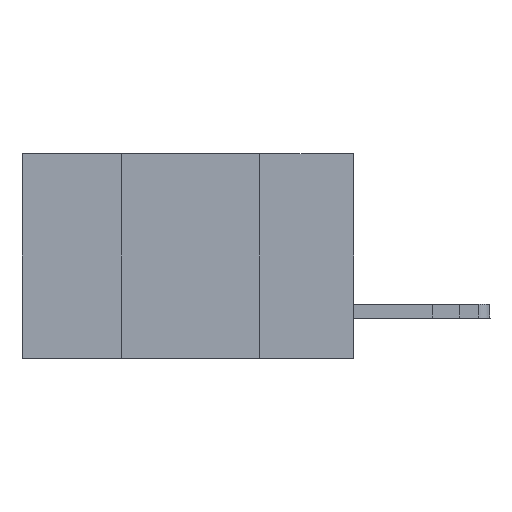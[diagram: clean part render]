
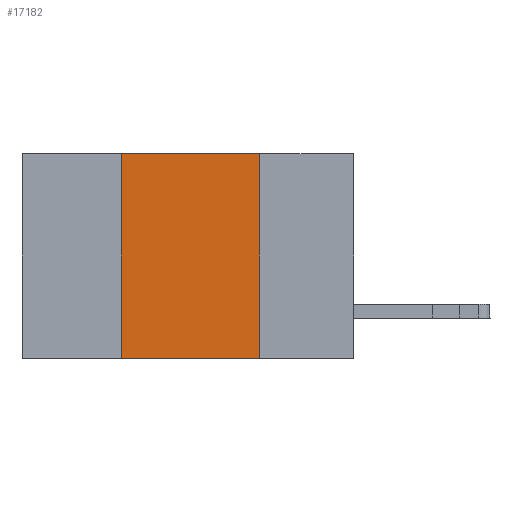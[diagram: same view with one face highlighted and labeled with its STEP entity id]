
A CAD part, left-side view. The second image highlights one B-rep face of the part: STEP entity #17182.
In plain terms, the highlighted planar face has unit normal (-1, 0, 0).
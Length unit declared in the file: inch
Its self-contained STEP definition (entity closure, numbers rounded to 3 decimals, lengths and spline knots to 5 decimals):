
#90 = CARTESIAN_POINT ( 'NONE',  ( 0., 0.42, 0. ) ) ;
#2150 = LINE ( 'NONE', #21750, #16067 ) ;
#2595 = DIRECTION ( 'NONE',  ( 0., -1., 0. ) ) ;
#3622 = ORIENTED_EDGE ( 'NONE', *, *, #23230, .F. ) ;
#3762 = AXIS2_PLACEMENT_3D ( 'NONE', #12570, #19631, #21415 ) ;
#4135 = ORIENTED_EDGE ( 'NONE', *, *, #12864, .F. ) ;
#4386 = VERTEX_POINT ( 'NONE', #21179 ) ;
#4761 = CARTESIAN_POINT ( 'NONE',  ( 0., 0.42, -0.37 ) ) ;
#5532 = DIRECTION ( 'NONE',  ( 0., 0., -1. ) ) ;
#6596 = LINE ( 'NONE', #8507, #18741 ) ;
#6712 = VERTEX_POINT ( 'NONE', #90 ) ;
#7334 = CARTESIAN_POINT ( 'NONE',  ( 0., 0.17, 0. ) ) ;
#8098 = LINE ( 'NONE', #17040, #13176 ) ;
#8507 = CARTESIAN_POINT ( 'NONE',  ( 0., 0.42, 0. ) ) ;
#8813 = VECTOR ( 'NONE', #5532, 39.37008 ) ;
#10406 = ORIENTED_EDGE ( 'NONE', *, *, #21756, .T. ) ;
#10437 = PLANE ( 'NONE',  #3762 ) ;
#11004 = ORIENTED_EDGE ( 'NONE', *, *, #22973, .F. ) ;
#11367 = EDGE_LOOP ( 'NONE', ( #11004, #4135, #3622, #10406 ) ) ;
#12065 = VERTEX_POINT ( 'NONE', #20813 ) ;
#12570 = CARTESIAN_POINT ( 'NONE',  ( 0., 0.6, 0. ) ) ;
#12864 = EDGE_CURVE ( 'NONE', #6712, #4386, #8098, .T. ) ;
#13176 = VECTOR ( 'NONE', #2595, 39.37008 ) ;
#13645 = VERTEX_POINT ( 'NONE', #4761 ) ;
#14236 = LINE ( 'NONE', #7334, #8813 ) ;
#14783 = DIRECTION ( 'NONE',  ( 0., -1., 0. ) ) ;
#16067 = VECTOR ( 'NONE', #14783, 39.37008 ) ;
#17040 = CARTESIAN_POINT ( 'NONE',  ( 0., 0.6, 0. ) ) ;
#17182 = ADVANCED_FACE ( 'NONE', ( #19986 ), #10437, .F. ) ;
#18741 = VECTOR ( 'NONE', #21170, 39.37008 ) ;
#19631 = DIRECTION ( 'NONE',  ( 1., 0., 0. ) ) ;
#19986 = FACE_OUTER_BOUND ( 'NONE', #11367, .T. ) ;
#20813 = CARTESIAN_POINT ( 'NONE',  ( 0., 0.17, -0.37 ) ) ;
#21170 = DIRECTION ( 'NONE',  ( 0., 0., 1. ) ) ;
#21179 = CARTESIAN_POINT ( 'NONE',  ( 0., 0.17, 0. ) ) ;
#21415 = DIRECTION ( 'NONE',  ( 0., 0., -1. ) ) ;
#21750 = CARTESIAN_POINT ( 'NONE',  ( 0., 0.6, -0.37 ) ) ;
#21756 = EDGE_CURVE ( 'NONE', #13645, #12065, #2150, .T. ) ;
#22973 = EDGE_CURVE ( 'NONE', #4386, #12065, #14236, .T. ) ;
#23230 = EDGE_CURVE ( 'NONE', #13645, #6712, #6596, .T. ) ;
